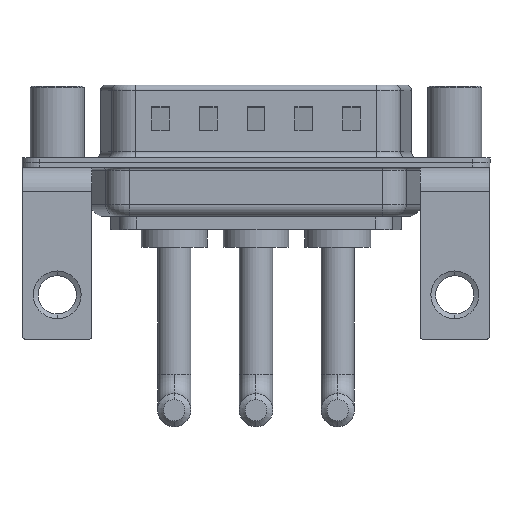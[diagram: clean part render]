
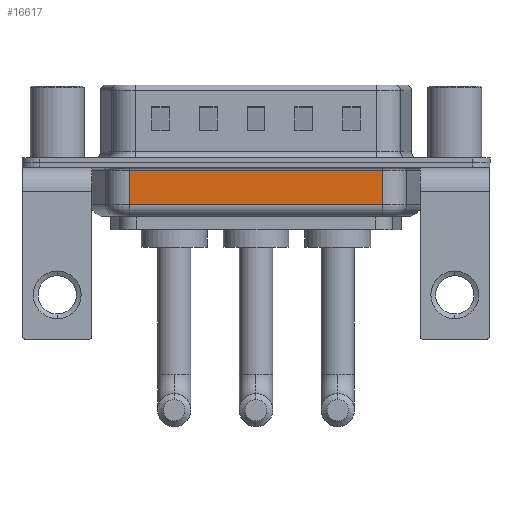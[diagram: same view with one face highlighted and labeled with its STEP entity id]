
A CAD part, front view. The second image highlights one B-rep face of the part: STEP entity #16617.
In plain terms, the highlighted planar face has unit normal (0, -1, 0).
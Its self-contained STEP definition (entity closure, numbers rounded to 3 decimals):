
#446 = CARTESIAN_POINT ( 'NONE',  ( 6.031, -5.35, -3.5 ) ) ;
#629 = CARTESIAN_POINT ( 'NONE',  ( 6.031, -5.35, -0.65 ) ) ;
#731 = ORIENTED_EDGE ( 'NONE', *, *, #2275, .F. ) ;
#1092 = EDGE_LOOP ( 'NONE', ( #731, #11983, #2508, #11587 ) ) ;
#1518 = VERTEX_POINT ( 'NONE', #12637 ) ;
#2251 = EDGE_CURVE ( 'NONE', #6456, #5396, #13074, .T. ) ;
#2275 = EDGE_CURVE ( 'NONE', #6456, #6803, #9851, .T. ) ;
#2447 = CARTESIAN_POINT ( 'NONE',  ( 27.269, -5.35, -4.5 ) ) ;
#2508 = ORIENTED_EDGE ( 'NONE', *, *, #8375, .T. ) ;
#2790 = CARTESIAN_POINT ( 'NONE',  ( 6.031, -5.35, -0.65 ) ) ;
#2829 = PLANE ( 'NONE',  #14450 ) ;
#3188 = CARTESIAN_POINT ( 'NONE',  ( 6.031, -5.35, -4.5 ) ) ;
#4258 = LINE ( 'NONE', #2790, #14673 ) ;
#4389 = DIRECTION ( 'NONE',  ( 0., 0., 1. ) ) ;
#5062 = CARTESIAN_POINT ( 'NONE',  ( 27.269, -5.35, -3.5 ) ) ;
#5318 = DIRECTION ( 'NONE',  ( 0., 1., 0. ) ) ;
#5396 = VERTEX_POINT ( 'NONE', #5062 ) ;
#5460 = DIRECTION ( 'NONE',  ( 0., 0., 1. ) ) ;
#5492 = CARTESIAN_POINT ( 'NONE',  ( 6.031, -5.35, -3.5 ) ) ;
#6456 = VERTEX_POINT ( 'NONE', #5492 ) ;
#6803 = VERTEX_POINT ( 'NONE', #629 ) ;
#6949 = VECTOR ( 'NONE', #5460, 1000. ) ;
#8272 = FACE_OUTER_BOUND ( 'NONE', #1092, .T. ) ;
#8375 = EDGE_CURVE ( 'NONE', #5396, #1518, #9627, .T. ) ;
#8859 = VECTOR ( 'NONE', #14360, 1000. ) ;
#9627 = LINE ( 'NONE', #2447, #6949 ) ;
#9766 = DIRECTION ( 'NONE',  ( 0., 0., 1. ) ) ;
#9851 = LINE ( 'NONE', #3188, #14778 ) ;
#11100 = DIRECTION ( 'NONE',  ( -1., 0., 0. ) ) ;
#11587 = ORIENTED_EDGE ( 'NONE', *, *, #13662, .T. ) ;
#11983 = ORIENTED_EDGE ( 'NONE', *, *, #2251, .T. ) ;
#12637 = CARTESIAN_POINT ( 'NONE',  ( 27.269, -5.35, -0.65 ) ) ;
#13074 = LINE ( 'NONE', #446, #8859 ) ;
#13662 = EDGE_CURVE ( 'NONE', #1518, #6803, #4258, .T. ) ;
#14004 = CARTESIAN_POINT ( 'NONE',  ( 6.031, -5.35, -4.5 ) ) ;
#14360 = DIRECTION ( 'NONE',  ( 1., 0., 0. ) ) ;
#14450 = AXIS2_PLACEMENT_3D ( 'NONE', #14004, #5318, #9766 ) ;
#14673 = VECTOR ( 'NONE', #11100, 1000. ) ;
#14778 = VECTOR ( 'NONE', #4389, 1000. ) ;
#16617 = ADVANCED_FACE ( 'NONE', ( #8272 ), #2829, .F. ) ;
